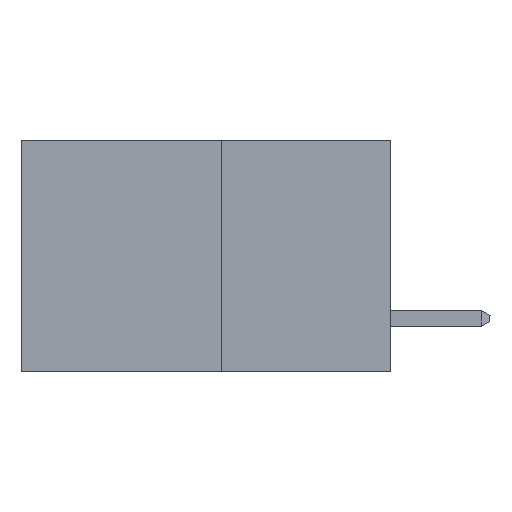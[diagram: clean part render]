
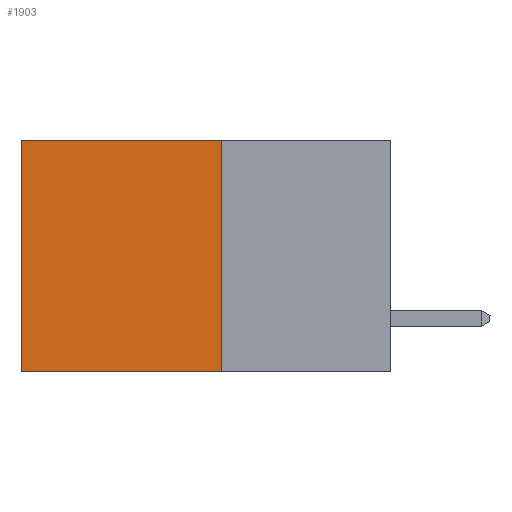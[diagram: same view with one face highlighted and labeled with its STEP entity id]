
A CAD part, left-side view. The second image highlights one B-rep face of the part: STEP entity #1903.
In plain terms, the highlighted planar face has unit normal (-1, 0, 0).
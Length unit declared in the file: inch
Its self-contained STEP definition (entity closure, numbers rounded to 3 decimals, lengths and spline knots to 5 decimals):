
#399 = VECTOR ( 'NONE', #8473, 39.37008 ) ;
#1049 = CARTESIAN_POINT ( 'NONE',  ( 0.277, 0.27, 0. ) ) ;
#1145 = DIRECTION ( 'NONE',  ( 0., 1., 0. ) ) ;
#1738 = EDGE_LOOP ( 'NONE', ( #8203, #7769, #10793, #2093 ) ) ;
#1850 = CARTESIAN_POINT ( 'NONE',  ( 0.277, 0.59, -0.37 ) ) ;
#1903 = ADVANCED_FACE ( 'NONE', ( #4157 ), #5621, .F. ) ;
#2093 = ORIENTED_EDGE ( 'NONE', *, *, #3869, .T. ) ;
#2483 = EDGE_CURVE ( 'NONE', #7603, #3791, #7394, .T. ) ;
#2718 = VERTEX_POINT ( 'NONE', #10249 ) ;
#3244 = DIRECTION ( 'NONE',  ( 0., 0., -1. ) ) ;
#3791 = VERTEX_POINT ( 'NONE', #1850 ) ;
#3869 = EDGE_CURVE ( 'NONE', #4419, #2718, #11135, .T. ) ;
#3967 = LINE ( 'NONE', #4414, #6012 ) ;
#4157 = FACE_OUTER_BOUND ( 'NONE', #1738, .T. ) ;
#4202 = CARTESIAN_POINT ( 'NONE',  ( 0.277, 0.27, 0. ) ) ;
#4414 = CARTESIAN_POINT ( 'NONE',  ( 0.277, 0.59, -0.37 ) ) ;
#4419 = VERTEX_POINT ( 'NONE', #4202 ) ;
#4526 = DIRECTION ( 'NONE',  ( 0., 0., -1. ) ) ;
#4637 = DIRECTION ( 'NONE',  ( 1., 0., 0. ) ) ;
#4919 = CARTESIAN_POINT ( 'NONE',  ( 0.277, 0.27, -0.37 ) ) ;
#5621 = PLANE ( 'NONE',  #6723 ) ;
#5753 = CARTESIAN_POINT ( 'NONE',  ( 0.277, 0.27, -0.37 ) ) ;
#6012 = VECTOR ( 'NONE', #9590, 39.37008 ) ;
#6110 = VECTOR ( 'NONE', #3244, 39.37008 ) ;
#6723 = AXIS2_PLACEMENT_3D ( 'NONE', #9528, #4637, #4526 ) ;
#7394 = LINE ( 'NONE', #5753, #399 ) ;
#7603 = VERTEX_POINT ( 'NONE', #4919 ) ;
#7647 = CARTESIAN_POINT ( 'NONE',  ( 0.277, 0.27, -0.37 ) ) ;
#7769 = ORIENTED_EDGE ( 'NONE', *, *, #2483, .F. ) ;
#7851 = EDGE_CURVE ( 'NONE', #2718, #3791, #3967, .T. ) ;
#8164 = LINE ( 'NONE', #7647, #6110 ) ;
#8203 = ORIENTED_EDGE ( 'NONE', *, *, #7851, .T. ) ;
#8473 = DIRECTION ( 'NONE',  ( 0., 1., 0. ) ) ;
#8705 = VECTOR ( 'NONE', #1145, 39.37008 ) ;
#9515 = EDGE_CURVE ( 'NONE', #4419, #7603, #8164, .T. ) ;
#9528 = CARTESIAN_POINT ( 'NONE',  ( 0.277, 0.27, -0.37 ) ) ;
#9590 = DIRECTION ( 'NONE',  ( 0., 0., -1. ) ) ;
#10249 = CARTESIAN_POINT ( 'NONE',  ( 0.277, 0.59, 0. ) ) ;
#10793 = ORIENTED_EDGE ( 'NONE', *, *, #9515, .F. ) ;
#11135 = LINE ( 'NONE', #1049, #8705 ) ;
